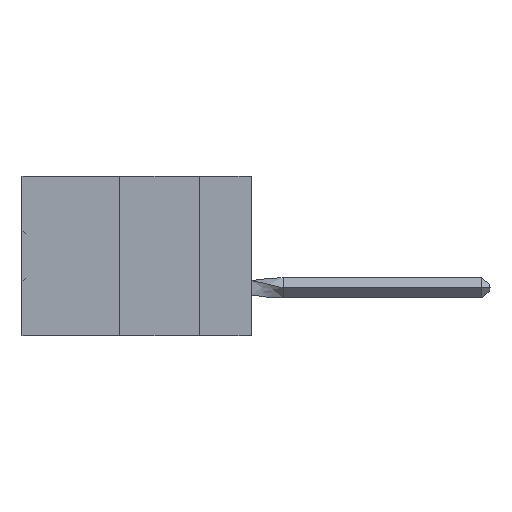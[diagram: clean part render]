
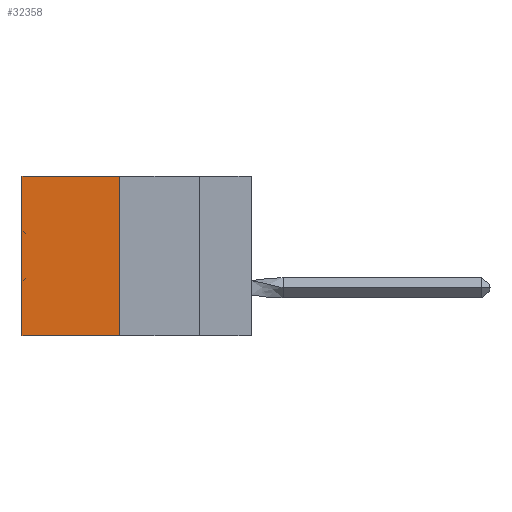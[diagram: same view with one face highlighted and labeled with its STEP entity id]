
A CAD part, left-side view. The second image highlights one B-rep face of the part: STEP entity #32358.
In plain terms, the highlighted planar face has unit normal (-1, 0, 0).
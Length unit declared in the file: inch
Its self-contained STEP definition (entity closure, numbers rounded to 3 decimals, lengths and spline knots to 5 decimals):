
#568 = DIRECTION ( 'NONE',  ( 0., 1., 0. ) ) ;
#650 = VERTEX_POINT ( 'NONE', #4964 ) ;
#1288 = DIRECTION ( 'NONE',  ( 0., 0., -1. ) ) ;
#1674 = EDGE_CURVE ( 'NONE', #15830, #650, #29522, .T. ) ;
#3751 = ORIENTED_EDGE ( 'NONE', *, *, #1674, .F. ) ;
#4964 = CARTESIAN_POINT ( 'NONE',  ( 0.305, 0.413, -0.5 ) ) ;
#5113 = CARTESIAN_POINT ( 'NONE',  ( 0.305, 0.413, 0. ) ) ;
#8616 = PLANE ( 'NONE',  #34089 ) ;
#9078 = VECTOR ( 'NONE', #568, 39.37008 ) ;
#10471 = ORIENTED_EDGE ( 'NONE', *, *, #17128, .F. ) ;
#10574 = VERTEX_POINT ( 'NONE', #43063 ) ;
#13303 = DIRECTION ( 'NONE',  ( 0., 0., -1. ) ) ;
#13764 = VECTOR ( 'NONE', #35589, 39.37008 ) ;
#15830 = VERTEX_POINT ( 'NONE', #29948 ) ;
#17128 = EDGE_CURVE ( 'NONE', #650, #10574, #20511, .T. ) ;
#20085 = ORIENTED_EDGE ( 'NONE', *, *, #49064, .T. ) ;
#20511 = LINE ( 'NONE', #31218, #9078 ) ;
#23120 = CARTESIAN_POINT ( 'NONE',  ( 0.305, 0.72, -0.5 ) ) ;
#24437 = FACE_OUTER_BOUND ( 'NONE', #50945, .T. ) ;
#26122 = CARTESIAN_POINT ( 'NONE',  ( 0.305, 0.413, -0.5 ) ) ;
#29273 = LINE ( 'NONE', #5113, #13764 ) ;
#29522 = LINE ( 'NONE', #26122, #30170 ) ;
#29948 = CARTESIAN_POINT ( 'NONE',  ( 0.305, 0.413, 0. ) ) ;
#30170 = VECTOR ( 'NONE', #43004, 39.37008 ) ;
#31218 = CARTESIAN_POINT ( 'NONE',  ( 0.305, 0.413, -0.5 ) ) ;
#32358 = ADVANCED_FACE ( 'NONE', ( #24437 ), #8616, .F. ) ;
#34089 = AXIS2_PLACEMENT_3D ( 'NONE', #42823, #34558, #13303 ) ;
#34558 = DIRECTION ( 'NONE',  ( 1., 0., 0. ) ) ;
#34607 = VECTOR ( 'NONE', #1288, 39.37008 ) ;
#35589 = DIRECTION ( 'NONE',  ( 0., 1., 0. ) ) ;
#38330 = ORIENTED_EDGE ( 'NONE', *, *, #47178, .T. ) ;
#39673 = CARTESIAN_POINT ( 'NONE',  ( 0.305, 0.72, 0. ) ) ;
#41092 = VERTEX_POINT ( 'NONE', #39673 ) ;
#42823 = CARTESIAN_POINT ( 'NONE',  ( 0.305, 0.413, -0.5 ) ) ;
#43004 = DIRECTION ( 'NONE',  ( 0., 0., -1. ) ) ;
#43063 = CARTESIAN_POINT ( 'NONE',  ( 0.305, 0.72, -0.5 ) ) ;
#47178 = EDGE_CURVE ( 'NONE', #41092, #10574, #54788, .T. ) ;
#49064 = EDGE_CURVE ( 'NONE', #15830, #41092, #29273, .T. ) ;
#50945 = EDGE_LOOP ( 'NONE', ( #38330, #10471, #3751, #20085 ) ) ;
#54788 = LINE ( 'NONE', #23120, #34607 ) ;
